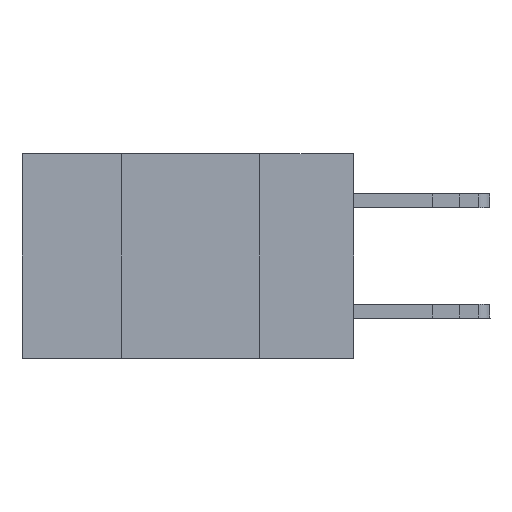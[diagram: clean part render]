
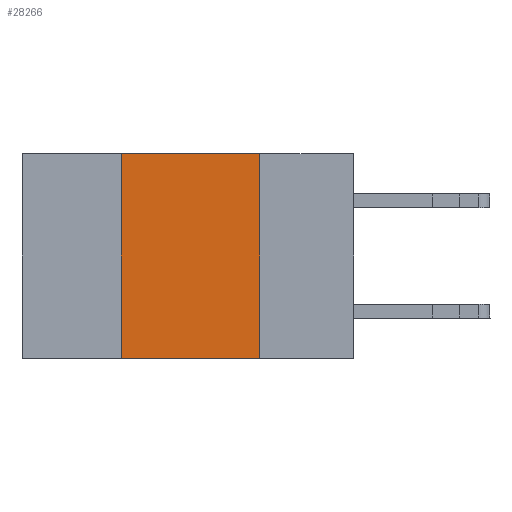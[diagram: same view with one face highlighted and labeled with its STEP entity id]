
A CAD part, left-side view. The second image highlights one B-rep face of the part: STEP entity #28266.
In plain terms, the highlighted planar face has unit normal (-1, 0, 0).
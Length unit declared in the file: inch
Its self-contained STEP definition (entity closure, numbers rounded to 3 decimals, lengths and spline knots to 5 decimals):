
#680 = VERTEX_POINT ( 'NONE', #14220 ) ;
#1749 = CARTESIAN_POINT ( 'NONE',  ( 0., 0.6, 0. ) ) ;
#2724 = CARTESIAN_POINT ( 'NONE',  ( 0., 0.42, -0.37 ) ) ;
#3921 = DIRECTION ( 'NONE',  ( 0., 0., -1. ) ) ;
#4915 = CARTESIAN_POINT ( 'NONE',  ( 0., 0.17, 0. ) ) ;
#5822 = VECTOR ( 'NONE', #21736, 39.37008 ) ;
#7928 = VERTEX_POINT ( 'NONE', #4915 ) ;
#8016 = DIRECTION ( 'NONE',  ( 0., -1., 0. ) ) ;
#8404 = VECTOR ( 'NONE', #3921, 39.37008 ) ;
#8574 = PLANE ( 'NONE',  #16503 ) ;
#10143 = CARTESIAN_POINT ( 'NONE',  ( 0., 0.6, 0. ) ) ;
#14130 = VECTOR ( 'NONE', #28042, 39.37008 ) ;
#14220 = CARTESIAN_POINT ( 'NONE',  ( 0., 0.17, -0.37 ) ) ;
#14578 = LINE ( 'NONE', #28031, #5822 ) ;
#14820 = ORIENTED_EDGE ( 'NONE', *, *, #15357, .T. ) ;
#15357 = EDGE_CURVE ( 'NONE', #22254, #680, #27323, .T. ) ;
#15813 = DIRECTION ( 'NONE',  ( 1., 0., 0. ) ) ;
#16082 = VECTOR ( 'NONE', #8016, 39.37008 ) ;
#16087 = CARTESIAN_POINT ( 'NONE',  ( 0., 0.6, -0.37 ) ) ;
#16175 = ORIENTED_EDGE ( 'NONE', *, *, #25429, .F. ) ;
#16503 = AXIS2_PLACEMENT_3D ( 'NONE', #1749, #15813, #29983 ) ;
#17958 = CARTESIAN_POINT ( 'NONE',  ( 0., 0.42, 0. ) ) ;
#19284 = EDGE_CURVE ( 'NONE', #26748, #7928, #23094, .T. ) ;
#19788 = EDGE_CURVE ( 'NONE', #22254, #26748, #14578, .T. ) ;
#21736 = DIRECTION ( 'NONE',  ( 0., 0., 1. ) ) ;
#22254 = VERTEX_POINT ( 'NONE', #2724 ) ;
#22426 = EDGE_LOOP ( 'NONE', ( #16175, #28811, #30276, #14820 ) ) ;
#23094 = LINE ( 'NONE', #10143, #16082 ) ;
#25429 = EDGE_CURVE ( 'NONE', #7928, #680, #27066, .T. ) ;
#26748 = VERTEX_POINT ( 'NONE', #17958 ) ;
#27066 = LINE ( 'NONE', #29487, #8404 ) ;
#27323 = LINE ( 'NONE', #16087, #14130 ) ;
#28031 = CARTESIAN_POINT ( 'NONE',  ( 0., 0.42, 0. ) ) ;
#28042 = DIRECTION ( 'NONE',  ( 0., -1., 0. ) ) ;
#28266 = ADVANCED_FACE ( 'NONE', ( #29334 ), #8574, .F. ) ;
#28811 = ORIENTED_EDGE ( 'NONE', *, *, #19284, .F. ) ;
#29334 = FACE_OUTER_BOUND ( 'NONE', #22426, .T. ) ;
#29487 = CARTESIAN_POINT ( 'NONE',  ( 0., 0.17, 0. ) ) ;
#29983 = DIRECTION ( 'NONE',  ( 0., 0., -1. ) ) ;
#30276 = ORIENTED_EDGE ( 'NONE', *, *, #19788, .F. ) ;
